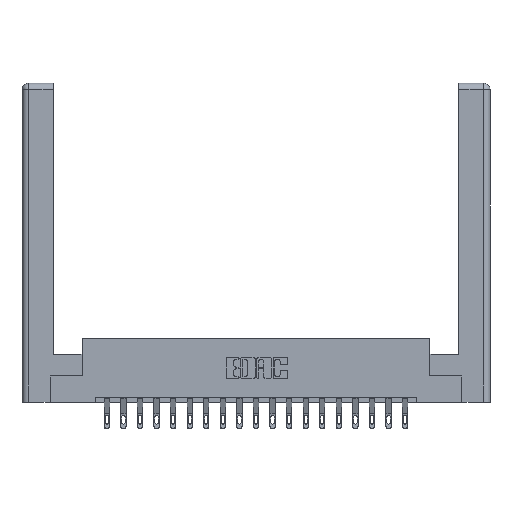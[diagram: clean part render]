
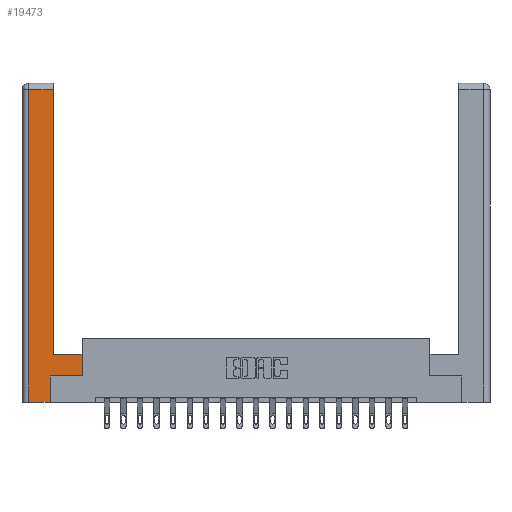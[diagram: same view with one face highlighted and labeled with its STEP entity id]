
A CAD part, top view. The second image highlights one B-rep face of the part: STEP entity #19473.
In plain terms, the highlighted planar face has unit normal (0, 0, 1).
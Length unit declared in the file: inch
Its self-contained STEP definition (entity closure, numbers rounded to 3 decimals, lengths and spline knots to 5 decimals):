
#15 = EDGE_CURVE ( 'NONE', #19719, #19102, #17105, .T. ) ;
#88 = CARTESIAN_POINT ( 'NONE',  ( 0.565, 0.45, 0. ) ) ;
#767 = EDGE_CURVE ( 'NONE', #20186, #19719, #4238, .T. ) ;
#1125 = DIRECTION ( 'NONE',  ( 0., 1., 0. ) ) ;
#1629 = VERTEX_POINT ( 'NONE', #4762 ) ;
#1924 = ORIENTED_EDGE ( 'NONE', *, *, #19076, .T. ) ;
#2252 = CARTESIAN_POINT ( 'NONE',  ( 0.295, 0.45, 0. ) ) ;
#2898 = DIRECTION ( 'NONE',  ( -1., 0., 0. ) ) ;
#2960 = EDGE_CURVE ( 'NONE', #3182, #20186, #13906, .T. ) ;
#3181 = VECTOR ( 'NONE', #3209, 39.37008 ) ;
#3182 = VERTEX_POINT ( 'NONE', #10155 ) ;
#3209 = DIRECTION ( 'NONE',  ( -1., 0., 0. ) ) ;
#3386 = ORIENTED_EDGE ( 'NONE', *, *, #2960, .T. ) ;
#4177 = CARTESIAN_POINT ( 'NONE',  ( 0.0615, 2.94, 0. ) ) ;
#4238 = LINE ( 'NONE', #14944, #13994 ) ;
#4239 = VECTOR ( 'NONE', #1125, 39.37008 ) ;
#4341 = CARTESIAN_POINT ( 'NONE',  ( 0.265, 0., 0. ) ) ;
#4762 = CARTESIAN_POINT ( 'NONE',  ( 0.265, 0.245, 0. ) ) ;
#5504 = CARTESIAN_POINT ( 'NONE',  ( 0.565, 0.245, 0. ) ) ;
#5567 = DIRECTION ( 'NONE',  ( 1., 0., 0. ) ) ;
#5701 = LINE ( 'NONE', #11153, #3181 ) ;
#5958 = DIRECTION ( 'NONE',  ( 0., 1., 0. ) ) ;
#6198 = LINE ( 'NONE', #5504, #18677 ) ;
#6809 = CARTESIAN_POINT ( 'NONE',  ( 0.265, 0., 0. ) ) ;
#6936 = DIRECTION ( 'NONE',  ( 0., -1., 0. ) ) ;
#7018 = CARTESIAN_POINT ( 'NONE',  ( 0., 0., 0. ) ) ;
#7175 = PLANE ( 'NONE',  #7805 ) ;
#7189 = VERTEX_POINT ( 'NONE', #10178 ) ;
#7236 = DIRECTION ( 'NONE',  ( -1., 0., 0. ) ) ;
#7293 = EDGE_LOOP ( 'NONE', ( #18984, #3386, #10159, #8315, #1924, #18997, #11600, #9760 ) ) ;
#7482 = LINE ( 'NONE', #16981, #10703 ) ;
#7805 = AXIS2_PLACEMENT_3D ( 'NONE', #7018, #8904, #7236 ) ;
#7925 = VECTOR ( 'NONE', #15671, 39.37008 ) ;
#8089 = VECTOR ( 'NONE', #8409, 39.37008 ) ;
#8315 = ORIENTED_EDGE ( 'NONE', *, *, #15, .T. ) ;
#8409 = DIRECTION ( 'NONE',  ( 1., 0., 0. ) ) ;
#8904 = DIRECTION ( 'NONE',  ( 0., 0., -1. ) ) ;
#9022 = EDGE_CURVE ( 'NONE', #15828, #3182, #10477, .T. ) ;
#9260 = CARTESIAN_POINT ( 'NONE',  ( 0.295, 3., 0. ) ) ;
#9760 = ORIENTED_EDGE ( 'NONE', *, *, #10466, .T. ) ;
#10021 = VERTEX_POINT ( 'NONE', #88 ) ;
#10155 = CARTESIAN_POINT ( 'NONE',  ( 0.295, 2.94, 0. ) ) ;
#10159 = ORIENTED_EDGE ( 'NONE', *, *, #767, .T. ) ;
#10178 = CARTESIAN_POINT ( 'NONE',  ( 0.565, 0.245, 0. ) ) ;
#10466 = EDGE_CURVE ( 'NONE', #10021, #15828, #5701, .T. ) ;
#10477 = LINE ( 'NONE', #9260, #4239 ) ;
#10703 = VECTOR ( 'NONE', #5958, 39.37008 ) ;
#11153 = CARTESIAN_POINT ( 'NONE',  ( 0.295, 0.45, 0. ) ) ;
#11600 = ORIENTED_EDGE ( 'NONE', *, *, #15544, .T. ) ;
#12178 = LINE ( 'NONE', #15803, #7925 ) ;
#12455 = CARTESIAN_POINT ( 'NONE',  ( 0.0615, 2.94, 0. ) ) ;
#13906 = LINE ( 'NONE', #12455, #14876 ) ;
#13994 = VECTOR ( 'NONE', #6936, 39.37008 ) ;
#14876 = VECTOR ( 'NONE', #2898, 39.37008 ) ;
#14944 = CARTESIAN_POINT ( 'NONE',  ( 0.0615, 0., 0. ) ) ;
#15297 = EDGE_CURVE ( 'NONE', #1629, #7189, #6198, .T. ) ;
#15544 = EDGE_CURVE ( 'NONE', #7189, #10021, #12178, .T. ) ;
#15671 = DIRECTION ( 'NONE',  ( 0., 1., 0. ) ) ;
#15803 = CARTESIAN_POINT ( 'NONE',  ( 0.565, 0.45, 0. ) ) ;
#15828 = VERTEX_POINT ( 'NONE', #2252 ) ;
#16981 = CARTESIAN_POINT ( 'NONE',  ( 0.265, 0.245, 0. ) ) ;
#17105 = LINE ( 'NONE', #6809, #8089 ) ;
#18252 = CARTESIAN_POINT ( 'NONE',  ( 0.0615, 0., 0. ) ) ;
#18677 = VECTOR ( 'NONE', #5567, 39.37008 ) ;
#18984 = ORIENTED_EDGE ( 'NONE', *, *, #9022, .T. ) ;
#18997 = ORIENTED_EDGE ( 'NONE', *, *, #15297, .T. ) ;
#19076 = EDGE_CURVE ( 'NONE', #19102, #1629, #7482, .T. ) ;
#19102 = VERTEX_POINT ( 'NONE', #4341 ) ;
#19457 = FACE_OUTER_BOUND ( 'NONE', #7293, .T. ) ;
#19473 = ADVANCED_FACE ( 'NONE', ( #19457 ), #7175, .F. ) ;
#19719 = VERTEX_POINT ( 'NONE', #18252 ) ;
#20186 = VERTEX_POINT ( 'NONE', #4177 ) ;
